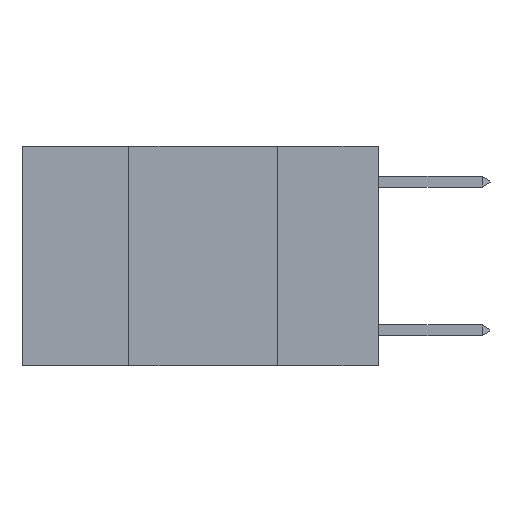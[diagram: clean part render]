
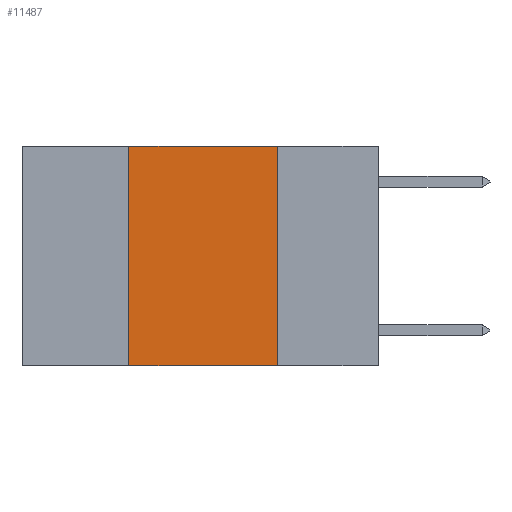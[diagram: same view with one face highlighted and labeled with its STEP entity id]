
A CAD part, left-side view. The second image highlights one B-rep face of the part: STEP entity #11487.
In plain terms, the highlighted planar face has unit normal (-1, 0, 0).
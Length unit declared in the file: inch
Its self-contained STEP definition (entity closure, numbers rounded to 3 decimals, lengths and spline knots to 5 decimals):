
#800 = AXIS2_PLACEMENT_3D ( 'NONE', #11841, #1231, #8743 ) ;
#1004 = LINE ( 'NONE', #8927, #7123 ) ;
#1092 = VERTEX_POINT ( 'NONE', #8480 ) ;
#1231 = DIRECTION ( 'NONE',  ( 1., 0., 0. ) ) ;
#1635 = DIRECTION ( 'NONE',  ( 0., 0., 1. ) ) ;
#1913 = ORIENTED_EDGE ( 'NONE', *, *, #10897, .F. ) ;
#1915 = EDGE_CURVE ( 'NONE', #1092, #12284, #1004, .T. ) ;
#1963 = VERTEX_POINT ( 'NONE', #9903 ) ;
#1989 = LINE ( 'NONE', #8076, #10484 ) ;
#2841 = DIRECTION ( 'NONE',  ( 0., -1., 0. ) ) ;
#2942 = VECTOR ( 'NONE', #10821, 39.37008 ) ;
#3482 = VECTOR ( 'NONE', #2841, 39.37008 ) ;
#3596 = CARTESIAN_POINT ( 'NONE',  ( 0., 0.42, 0. ) ) ;
#4102 = EDGE_CURVE ( 'NONE', #1092, #10678, #1989, .T. ) ;
#4478 = PLANE ( 'NONE',  #800 ) ;
#6119 = ORIENTED_EDGE ( 'NONE', *, *, #1915, .T. ) ;
#6238 = EDGE_LOOP ( 'NONE', ( #9765, #1913, #11047, #6119 ) ) ;
#6324 = LINE ( 'NONE', #7118, #3482 ) ;
#7118 = CARTESIAN_POINT ( 'NONE',  ( 0., 0.6, 0. ) ) ;
#7123 = VECTOR ( 'NONE', #9939, 39.37008 ) ;
#7487 = FACE_OUTER_BOUND ( 'NONE', #6238, .T. ) ;
#8076 = CARTESIAN_POINT ( 'NONE',  ( 0., 0.42, 0. ) ) ;
#8480 = CARTESIAN_POINT ( 'NONE',  ( 0., 0.42, -0.37 ) ) ;
#8607 = LINE ( 'NONE', #9785, #2942 ) ;
#8743 = DIRECTION ( 'NONE',  ( 0., 0., -1. ) ) ;
#8927 = CARTESIAN_POINT ( 'NONE',  ( 0., 0.6, -0.37 ) ) ;
#9765 = ORIENTED_EDGE ( 'NONE', *, *, #12135, .F. ) ;
#9785 = CARTESIAN_POINT ( 'NONE',  ( 0., 0.17, 0. ) ) ;
#9903 = CARTESIAN_POINT ( 'NONE',  ( 0., 0.17, 0. ) ) ;
#9939 = DIRECTION ( 'NONE',  ( 0., -1., 0. ) ) ;
#10007 = CARTESIAN_POINT ( 'NONE',  ( 0., 0.17, -0.37 ) ) ;
#10484 = VECTOR ( 'NONE', #1635, 39.37008 ) ;
#10678 = VERTEX_POINT ( 'NONE', #3596 ) ;
#10821 = DIRECTION ( 'NONE',  ( 0., 0., -1. ) ) ;
#10897 = EDGE_CURVE ( 'NONE', #10678, #1963, #6324, .T. ) ;
#11047 = ORIENTED_EDGE ( 'NONE', *, *, #4102, .F. ) ;
#11487 = ADVANCED_FACE ( 'NONE', ( #7487 ), #4478, .F. ) ;
#11841 = CARTESIAN_POINT ( 'NONE',  ( 0., 0.6, 0. ) ) ;
#12135 = EDGE_CURVE ( 'NONE', #1963, #12284, #8607, .T. ) ;
#12284 = VERTEX_POINT ( 'NONE', #10007 ) ;
